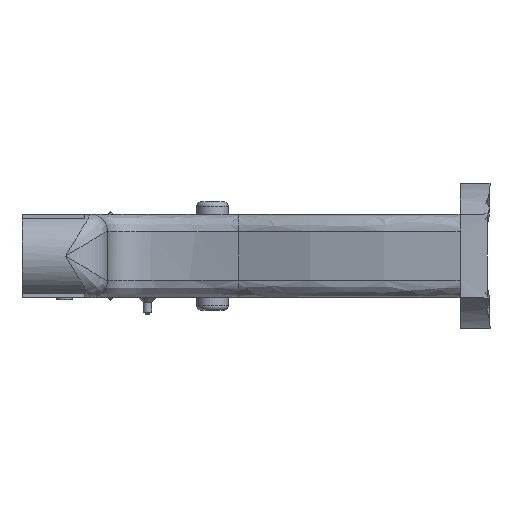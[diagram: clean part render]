
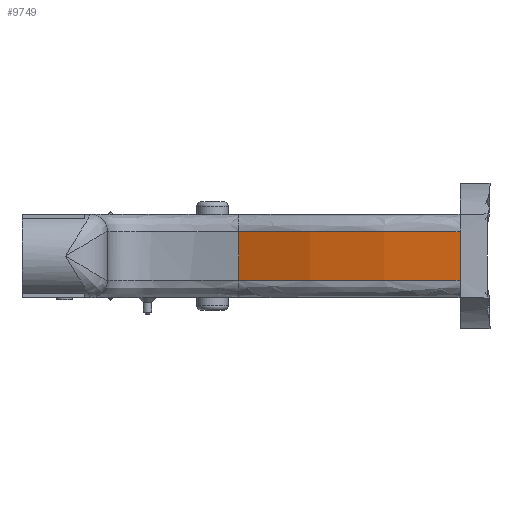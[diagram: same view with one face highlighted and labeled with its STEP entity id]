
A CAD part, left-side view. The second image highlights one B-rep face of the part: STEP entity #9749.
In plain terms, the highlighted cylindrical face has radius 144.148 mm (diameter 288.295 mm), a partial arc.
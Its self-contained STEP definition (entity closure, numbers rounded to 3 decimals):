
#208=CYLINDRICAL_SURFACE('',#10439,144.148);
#508=CIRCLE('',#10437,144.148);
#509=CIRCLE('',#10438,144.148);
#1343=FACE_OUTER_BOUND('',#1889,.T.);
#1889=EDGE_LOOP('',(#8863,#8864,#8865,#8866));
#2267=LINE('',#16355,#3136);
#2713=LINE('',#24418,#3582);
#3136=VECTOR('',#11158,10.);
#3582=VECTOR('',#12476,10.);
#4140=VERTEX_POINT('',#16341);
#4141=VERTEX_POINT('',#16354);
#4579=VERTEX_POINT('',#24267);
#4580=VERTEX_POINT('',#24397);
#5195=EDGE_CURVE('',#4140,#4141,#2267,.T.);
#5975=EDGE_CURVE('',#4580,#4579,#2713,.T.);
#6046=EDGE_CURVE('',#4579,#4141,#508,.T.);
#6047=EDGE_CURVE('',#4580,#4140,#509,.T.);
#8863=ORIENTED_EDGE('',*,*,#5195,.F.);
#8864=ORIENTED_EDGE('',*,*,#6047,.F.);
#8865=ORIENTED_EDGE('',*,*,#5975,.T.);
#8866=ORIENTED_EDGE('',*,*,#6046,.T.);
#9749=ADVANCED_FACE('',(#1343),#208,.T.);
#10437=AXIS2_PLACEMENT_3D('',#24799,#12657,#12658);
#10438=AXIS2_PLACEMENT_3D('',#24836,#12659,#12660);
#10439=AXIS2_PLACEMENT_3D('',#24837,#12661,#12662);
#11158=DIRECTION('',(0.,0.,-1.));
#12476=DIRECTION('',(0.,0.,-1.));
#12657=DIRECTION('center_axis',(0.,0.,
1.));
#12658=DIRECTION('ref_axis',(-0.899,0.437,0.));
#12659=DIRECTION('center_axis',(0.,0.,1.));
#12660=DIRECTION('ref_axis',(-0.899,0.437,0.));
#12661=DIRECTION('center_axis',(0.,0.,
1.));
#12662=DIRECTION('ref_axis',(-0.893,0.45,0.));
#16341=CARTESIAN_POINT('',(-82.277,-57.79,23.28));
#16354=CARTESIAN_POINT('',(-82.277,-57.79,11.72));
#16355=CARTESIAN_POINT('',(-82.277,-57.79,17.5));
#24267=CARTESIAN_POINT('',(-68.113,-4.565,11.72));
#24397=CARTESIAN_POINT('',(-68.113,-4.565,23.28));
#24418=CARTESIAN_POINT('',(-68.113,-4.565,27.5));
#24799=CARTESIAN_POINT('Origin',(61.539,-67.563,11.72));
#24836=CARTESIAN_POINT('Origin',(61.539,-67.563,23.28));
#24837=CARTESIAN_POINT('Origin',(61.539,-67.563,17.5));
